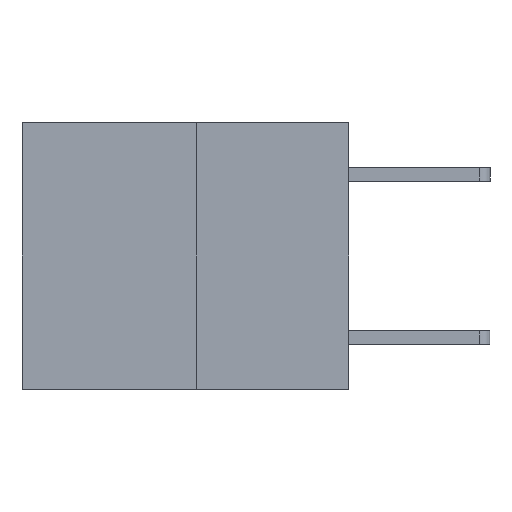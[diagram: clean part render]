
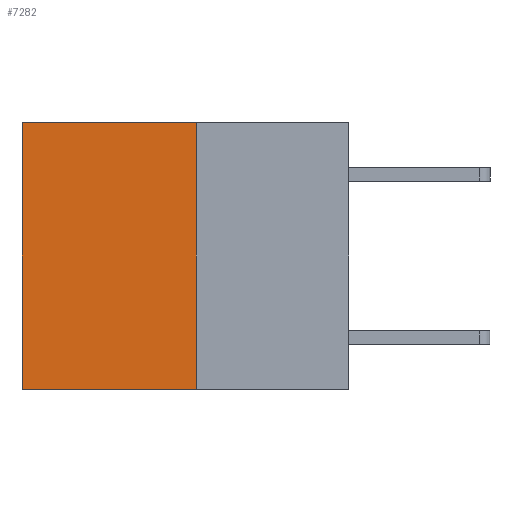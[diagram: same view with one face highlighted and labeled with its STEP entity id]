
A CAD part, left-side view. The second image highlights one B-rep face of the part: STEP entity #7282.
In plain terms, the highlighted planar face has unit normal (-1, 0, 0).
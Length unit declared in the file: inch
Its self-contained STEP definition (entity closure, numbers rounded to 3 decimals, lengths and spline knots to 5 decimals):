
#216 = EDGE_CURVE ( 'NONE', #491, #5649, #6635, .T. ) ;
#219 = VECTOR ( 'NONE', #7782, 39.37008 ) ;
#491 = VERTEX_POINT ( 'NONE', #4087 ) ;
#750 = CARTESIAN_POINT ( 'NONE',  ( 0.3165, 0.28, -0.49 ) ) ;
#815 = CARTESIAN_POINT ( 'NONE',  ( 0.3165, 0.6, -0.49 ) ) ;
#1242 = EDGE_LOOP ( 'NONE', ( #2320, #6787, #1872, #6419 ) ) ;
#1303 = LINE ( 'NONE', #6674, #7635 ) ;
#1455 = VECTOR ( 'NONE', #4661, 39.37008 ) ;
#1523 = DIRECTION ( 'NONE',  ( 0., 0., -1. ) ) ;
#1872 = ORIENTED_EDGE ( 'NONE', *, *, #5059, .F. ) ;
#2320 = ORIENTED_EDGE ( 'NONE', *, *, #216, .T. ) ;
#2446 = CARTESIAN_POINT ( 'NONE',  ( 0.3165, 0.28, 0. ) ) ;
#2558 = FACE_OUTER_BOUND ( 'NONE', #1242, .T. ) ;
#2703 = AXIS2_PLACEMENT_3D ( 'NONE', #5374, #2765, #1523 ) ;
#2765 = DIRECTION ( 'NONE',  ( 1., 0., 0. ) ) ;
#3185 = LINE ( 'NONE', #7730, #1455 ) ;
#3759 = VECTOR ( 'NONE', #5142, 39.37008 ) ;
#4087 = CARTESIAN_POINT ( 'NONE',  ( 0.3165, 0.6, 0. ) ) ;
#4292 = EDGE_CURVE ( 'NONE', #4969, #5649, #5044, .T. ) ;
#4522 = CARTESIAN_POINT ( 'NONE',  ( 0.3165, 0.6, -0.49 ) ) ;
#4661 = DIRECTION ( 'NONE',  ( 0., 0., -1. ) ) ;
#4969 = VERTEX_POINT ( 'NONE', #750 ) ;
#5044 = LINE ( 'NONE', #5329, #219 ) ;
#5059 = EDGE_CURVE ( 'NONE', #5442, #4969, #3185, .T. ) ;
#5142 = DIRECTION ( 'NONE',  ( 0., 0., -1. ) ) ;
#5329 = CARTESIAN_POINT ( 'NONE',  ( 0.3165, 0.28, -0.49 ) ) ;
#5374 = CARTESIAN_POINT ( 'NONE',  ( 0.3165, 0.28, -0.49 ) ) ;
#5418 = PLANE ( 'NONE',  #2703 ) ;
#5442 = VERTEX_POINT ( 'NONE', #2446 ) ;
#5649 = VERTEX_POINT ( 'NONE', #815 ) ;
#6419 = ORIENTED_EDGE ( 'NONE', *, *, #7439, .T. ) ;
#6635 = LINE ( 'NONE', #4522, #3759 ) ;
#6674 = CARTESIAN_POINT ( 'NONE',  ( 0.3165, 0.28, 0. ) ) ;
#6776 = DIRECTION ( 'NONE',  ( 0., 1., 0. ) ) ;
#6787 = ORIENTED_EDGE ( 'NONE', *, *, #4292, .F. ) ;
#7282 = ADVANCED_FACE ( 'NONE', ( #2558 ), #5418, .F. ) ;
#7439 = EDGE_CURVE ( 'NONE', #5442, #491, #1303, .T. ) ;
#7635 = VECTOR ( 'NONE', #6776, 39.37008 ) ;
#7730 = CARTESIAN_POINT ( 'NONE',  ( 0.3165, 0.28, -0.49 ) ) ;
#7782 = DIRECTION ( 'NONE',  ( 0., 1., 0. ) ) ;
